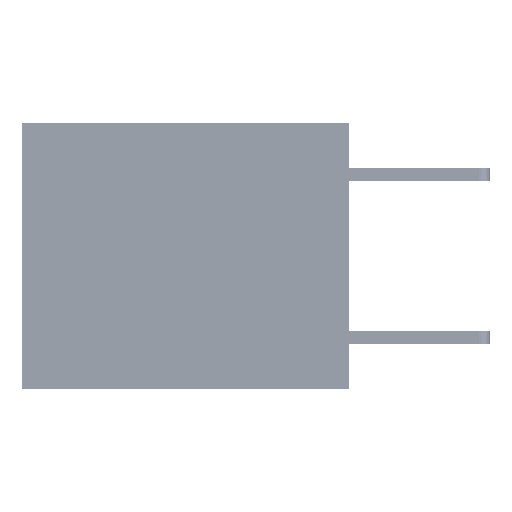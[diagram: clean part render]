
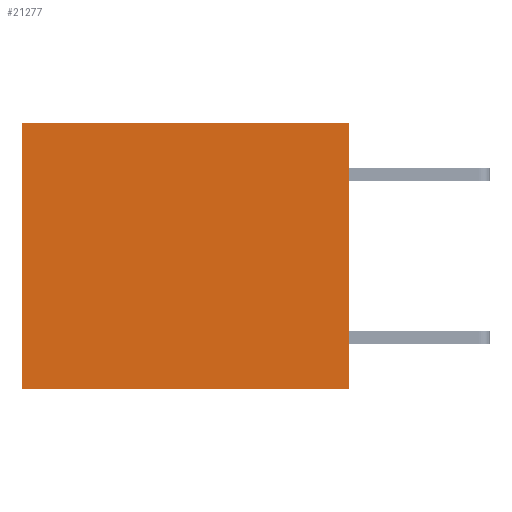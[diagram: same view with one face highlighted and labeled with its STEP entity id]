
A CAD part, left-side view. The second image highlights one B-rep face of the part: STEP entity #21277.
In plain terms, the highlighted planar face has unit normal (-1, 0, 0).
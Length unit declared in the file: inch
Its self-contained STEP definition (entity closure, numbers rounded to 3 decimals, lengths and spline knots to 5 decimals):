
#3494 = LINE ( 'NONE', #23704, #24887 ) ;
#3727 = VERTEX_POINT ( 'NONE', #32646 ) ;
#4081 = EDGE_CURVE ( 'NONE', #5059, #17585, #5583, .T. ) ;
#5059 = VERTEX_POINT ( 'NONE', #22834 ) ;
#5279 = CARTESIAN_POINT ( 'NONE',  ( 0.3165, 0., 0. ) ) ;
#5583 = LINE ( 'NONE', #6635, #11107 ) ;
#6035 = ORIENTED_EDGE ( 'NONE', *, *, #4081, .T. ) ;
#6332 = VECTOR ( 'NONE', #8135, 39.37008 ) ;
#6635 = CARTESIAN_POINT ( 'NONE',  ( 0.3165, 0.6, -0.49 ) ) ;
#6829 = CARTESIAN_POINT ( 'NONE',  ( 0.3165, 0.6, -0.49 ) ) ;
#7355 = EDGE_LOOP ( 'NONE', ( #6035, #12703, #25573, #12806 ) ) ;
#8135 = DIRECTION ( 'NONE',  ( 0., 1., 0. ) ) ;
#9132 = EDGE_CURVE ( 'NONE', #16738, #17585, #26989, .T. ) ;
#9215 = DIRECTION ( 'NONE',  ( 1., 0., 0. ) ) ;
#11077 = DIRECTION ( 'NONE',  ( 0., 1., 0. ) ) ;
#11107 = VECTOR ( 'NONE', #12189, 39.37008 ) ;
#12189 = DIRECTION ( 'NONE',  ( 0., 0., -1. ) ) ;
#12678 = LINE ( 'NONE', #5279, #6332 ) ;
#12703 = ORIENTED_EDGE ( 'NONE', *, *, #9132, .F. ) ;
#12806 = ORIENTED_EDGE ( 'NONE', *, *, #25638, .T. ) ;
#14905 = VECTOR ( 'NONE', #11077, 39.37008 ) ;
#15049 = DIRECTION ( 'NONE',  ( 0., 0., -1. ) ) ;
#16689 = CARTESIAN_POINT ( 'NONE',  ( 0.3165, 0., -0.49 ) ) ;
#16738 = VERTEX_POINT ( 'NONE', #17648 ) ;
#17585 = VERTEX_POINT ( 'NONE', #6829 ) ;
#17648 = CARTESIAN_POINT ( 'NONE',  ( 0.3165, 0., -0.49 ) ) ;
#17664 = FACE_OUTER_BOUND ( 'NONE', #7355, .T. ) ;
#21277 = ADVANCED_FACE ( 'NONE', ( #17664 ), #28790, .F. ) ;
#22834 = CARTESIAN_POINT ( 'NONE',  ( 0.3165, 0.6, 0. ) ) ;
#22968 = AXIS2_PLACEMENT_3D ( 'NONE', #25647, #9215, #15049 ) ;
#23704 = CARTESIAN_POINT ( 'NONE',  ( 0.3165, 0., -0.49 ) ) ;
#24440 = DIRECTION ( 'NONE',  ( 0., 0., -1. ) ) ;
#24887 = VECTOR ( 'NONE', #24440, 39.37008 ) ;
#25573 = ORIENTED_EDGE ( 'NONE', *, *, #28934, .F. ) ;
#25638 = EDGE_CURVE ( 'NONE', #3727, #5059, #12678, .T. ) ;
#25647 = CARTESIAN_POINT ( 'NONE',  ( 0.3165, 0., -0.49 ) ) ;
#26989 = LINE ( 'NONE', #16689, #14905 ) ;
#28790 = PLANE ( 'NONE',  #22968 ) ;
#28934 = EDGE_CURVE ( 'NONE', #3727, #16738, #3494, .T. ) ;
#32646 = CARTESIAN_POINT ( 'NONE',  ( 0.3165, 0., 0. ) ) ;
